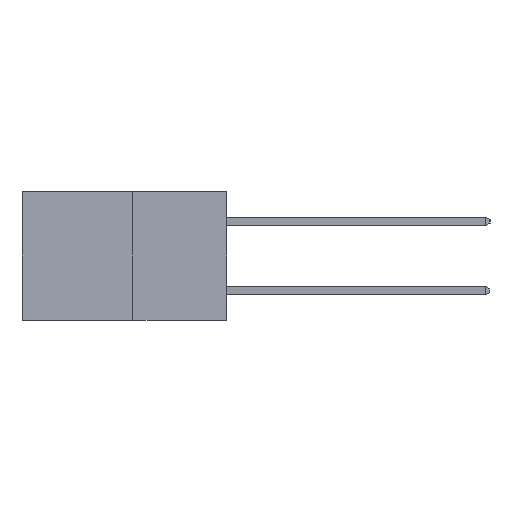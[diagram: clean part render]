
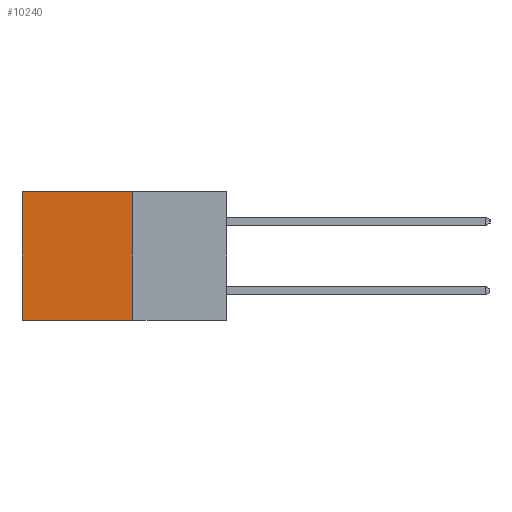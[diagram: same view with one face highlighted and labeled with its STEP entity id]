
A CAD part, left-side view. The second image highlights one B-rep face of the part: STEP entity #10240.
In plain terms, the highlighted planar face has unit normal (-1, 0, 0).
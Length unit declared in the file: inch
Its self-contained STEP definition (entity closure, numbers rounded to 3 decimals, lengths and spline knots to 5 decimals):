
#168 = VECTOR ( 'NONE', #14573, 39.37008 ) ;
#398 = DIRECTION ( 'NONE',  ( 1., 0., 0. ) ) ;
#886 = VECTOR ( 'NONE', #15792, 39.37008 ) ;
#1646 = VECTOR ( 'NONE', #11625, 39.37008 ) ;
#1742 = CARTESIAN_POINT ( 'NONE',  ( 0.277, 0.59, 0. ) ) ;
#1881 = CARTESIAN_POINT ( 'NONE',  ( 0.277, 0.27, -0.37 ) ) ;
#2354 = DIRECTION ( 'NONE',  ( 0., 0., -1. ) ) ;
#3743 = AXIS2_PLACEMENT_3D ( 'NONE', #12851, #398, #10199 ) ;
#3958 = EDGE_CURVE ( 'NONE', #17612, #8022, #7579, .T. ) ;
#4088 = EDGE_CURVE ( 'NONE', #5141, #17612, #5370, .T. ) ;
#4460 = ORIENTED_EDGE ( 'NONE', *, *, #3958, .T. ) ;
#5141 = VERTEX_POINT ( 'NONE', #13731 ) ;
#5370 = LINE ( 'NONE', #11684, #1646 ) ;
#7578 = ORIENTED_EDGE ( 'NONE', *, *, #4088, .T. ) ;
#7579 = LINE ( 'NONE', #14255, #168 ) ;
#8022 = VERTEX_POINT ( 'NONE', #9849 ) ;
#9849 = CARTESIAN_POINT ( 'NONE',  ( 0.277, 0.59, -0.37 ) ) ;
#9854 = VECTOR ( 'NONE', #2354, 39.37008 ) ;
#10199 = DIRECTION ( 'NONE',  ( 0., 0., -1. ) ) ;
#10216 = VERTEX_POINT ( 'NONE', #12913 ) ;
#10240 = ADVANCED_FACE ( 'NONE', ( #16561 ), #15632, .F. ) ;
#10720 = LINE ( 'NONE', #12155, #9854 ) ;
#11625 = DIRECTION ( 'NONE',  ( 0., 1., 0. ) ) ;
#11684 = CARTESIAN_POINT ( 'NONE',  ( 0.277, 0.27, 0. ) ) ;
#12155 = CARTESIAN_POINT ( 'NONE',  ( 0.277, 0.27, -0.37 ) ) ;
#12198 = ORIENTED_EDGE ( 'NONE', *, *, #17836, .F. ) ;
#12680 = ORIENTED_EDGE ( 'NONE', *, *, #16902, .F. ) ;
#12851 = CARTESIAN_POINT ( 'NONE',  ( 0.277, 0.27, -0.37 ) ) ;
#12913 = CARTESIAN_POINT ( 'NONE',  ( 0.277, 0.27, -0.37 ) ) ;
#13731 = CARTESIAN_POINT ( 'NONE',  ( 0.277, 0.27, 0. ) ) ;
#14255 = CARTESIAN_POINT ( 'NONE',  ( 0.277, 0.59, -0.37 ) ) ;
#14573 = DIRECTION ( 'NONE',  ( 0., 0., -1. ) ) ;
#15632 = PLANE ( 'NONE',  #3743 ) ;
#15671 = LINE ( 'NONE', #1881, #886 ) ;
#15792 = DIRECTION ( 'NONE',  ( 0., 1., 0. ) ) ;
#16561 = FACE_OUTER_BOUND ( 'NONE', #17721, .T. ) ;
#16902 = EDGE_CURVE ( 'NONE', #10216, #8022, #15671, .T. ) ;
#17612 = VERTEX_POINT ( 'NONE', #1742 ) ;
#17721 = EDGE_LOOP ( 'NONE', ( #4460, #12680, #12198, #7578 ) ) ;
#17836 = EDGE_CURVE ( 'NONE', #5141, #10216, #10720, .T. ) ;
